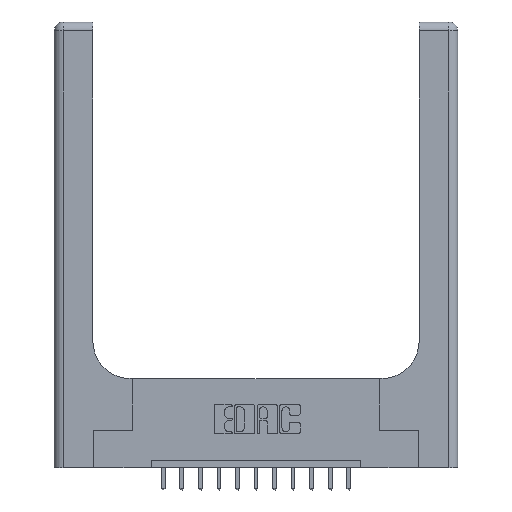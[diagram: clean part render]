
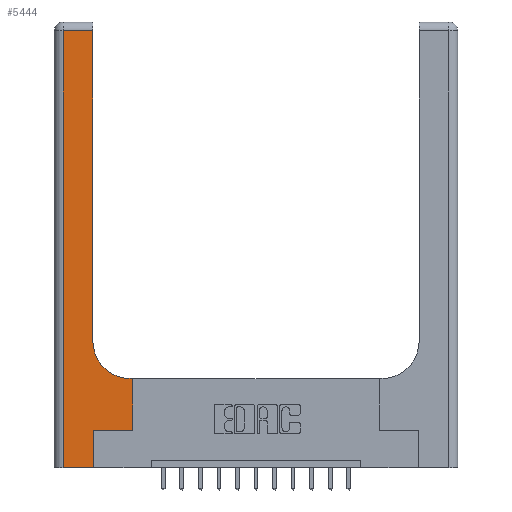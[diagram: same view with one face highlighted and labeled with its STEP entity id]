
A CAD part, top view. The second image highlights one B-rep face of the part: STEP entity #5444.
In plain terms, the highlighted planar face has unit normal (0, 0, 1).
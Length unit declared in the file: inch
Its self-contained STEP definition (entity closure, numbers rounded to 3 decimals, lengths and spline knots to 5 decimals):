
#220 = CARTESIAN_POINT ( 'NONE',  ( 0.51, 0.85, 0.37 ) ) ;
#249 = LINE ( 'NONE', #14911, #7896 ) ;
#260 = DIRECTION ( 'NONE',  ( 0., -1., 0. ) ) ;
#289 = VECTOR ( 'NONE', #5179, 39.37008 ) ;
#302 = DIRECTION ( 'NONE',  ( 0., 0., -1. ) ) ;
#724 = EDGE_CURVE ( 'NONE', #6429, #13446, #13874, .T. ) ;
#1127 = VERTEX_POINT ( 'NONE', #4149 ) ;
#1503 = VECTOR ( 'NONE', #8456, 39.37008 ) ;
#1571 = CARTESIAN_POINT ( 'NONE',  ( 0.528, 0.25, 0.37 ) ) ;
#1574 = CARTESIAN_POINT ( 'NONE',  ( 0.06, 0., 0.37 ) ) ;
#1593 = DIRECTION ( 'NONE',  ( 0., 0., -1. ) ) ;
#1599 = ORIENTED_EDGE ( 'NONE', *, *, #724, .T. ) ;
#1670 = FACE_OUTER_BOUND ( 'NONE', #6649, .T. ) ;
#1746 = VECTOR ( 'NONE', #3980, 39.37008 ) ;
#2108 = EDGE_CURVE ( 'NONE', #6239, #6429, #3733, .T. ) ;
#2227 = CARTESIAN_POINT ( 'NONE',  ( 0., 0., 0.37 ) ) ;
#2415 = VECTOR ( 'NONE', #10164, 39.37008 ) ;
#2502 = CARTESIAN_POINT ( 'NONE',  ( 0.26, 0.85, 0.37 ) ) ;
#2815 = VECTOR ( 'NONE', #260, 39.37008 ) ;
#3072 = DIRECTION ( 'NONE',  ( 1., 0., 0. ) ) ;
#3111 = DIRECTION ( 'NONE',  ( -1., 0., 0. ) ) ;
#3733 = LINE ( 'NONE', #10116, #4540 ) ;
#3980 = DIRECTION ( 'NONE',  ( 1., 0., 0. ) ) ;
#3993 = EDGE_CURVE ( 'NONE', #7947, #6239, #6394, .T. ) ;
#4127 = VERTEX_POINT ( 'NONE', #6884 ) ;
#4149 = CARTESIAN_POINT ( 'NONE',  ( 0.51, 0.6, 0.37 ) ) ;
#4290 = PLANE ( 'NONE',  #7903 ) ;
#4540 = VECTOR ( 'NONE', #7610, 39.37008 ) ;
#5090 = ORIENTED_EDGE ( 'NONE', *, *, #14723, .T. ) ;
#5179 = DIRECTION ( 'NONE',  ( 0., 1., 0. ) ) ;
#5444 = ADVANCED_FACE ( 'NONE', ( #1670 ), #4290, .F. ) ;
#5462 = EDGE_CURVE ( 'NONE', #8586, #14287, #6637, .T. ) ;
#5577 = DIRECTION ( 'NONE',  ( 0., 1., 0. ) ) ;
#5618 = ORIENTED_EDGE ( 'NONE', *, *, #2108, .T. ) ;
#6239 = VERTEX_POINT ( 'NONE', #7311 ) ;
#6394 = LINE ( 'NONE', #15412, #2415 ) ;
#6429 = VERTEX_POINT ( 'NONE', #1571 ) ;
#6637 = LINE ( 'NONE', #6725, #2815 ) ;
#6649 = EDGE_LOOP ( 'NONE', ( #9048, #15503, #15206, #15675, #10829, #5618, #1599, #8848, #5090 ) ) ;
#6706 = EDGE_CURVE ( 'NONE', #4127, #8586, #7115, .T. ) ;
#6725 = CARTESIAN_POINT ( 'NONE',  ( 0.06, 3., 0.37 ) ) ;
#6884 = CARTESIAN_POINT ( 'NONE',  ( 0.26, 2.94, 0.37 ) ) ;
#7115 = LINE ( 'NONE', #11091, #1503 ) ;
#7143 = AXIS2_PLACEMENT_3D ( 'NONE', #220, #302, #3072 ) ;
#7311 = CARTESIAN_POINT ( 'NONE',  ( 0.265, 0.25, 0.37 ) ) ;
#7610 = DIRECTION ( 'NONE',  ( 1., 0., 0. ) ) ;
#7896 = VECTOR ( 'NONE', #12388, 39.37008 ) ;
#7903 = AXIS2_PLACEMENT_3D ( 'NONE', #10757, #1593, #3111 ) ;
#7947 = VERTEX_POINT ( 'NONE', #16629 ) ;
#8456 = DIRECTION ( 'NONE',  ( -1., 0., 0. ) ) ;
#8586 = VERTEX_POINT ( 'NONE', #12579 ) ;
#8607 = LINE ( 'NONE', #2227, #1746 ) ;
#8848 = ORIENTED_EDGE ( 'NONE', *, *, #11208, .T. ) ;
#9048 = ORIENTED_EDGE ( 'NONE', *, *, #16165, .T. ) ;
#10116 = CARTESIAN_POINT ( 'NONE',  ( 0.265, 0.25, 0.37 ) ) ;
#10164 = DIRECTION ( 'NONE',  ( 0., 1., 0. ) ) ;
#10443 = LINE ( 'NONE', #11980, #14202 ) ;
#10630 = CIRCLE ( 'NONE', #7143, 0.25 ) ;
#10757 = CARTESIAN_POINT ( 'NONE',  ( 0., 3., 0.37 ) ) ;
#10829 = ORIENTED_EDGE ( 'NONE', *, *, #3993, .T. ) ;
#11091 = CARTESIAN_POINT ( 'NONE',  ( 0., 2.94, 0.37 ) ) ;
#11208 = EDGE_CURVE ( 'NONE', #13446, #1127, #249, .T. ) ;
#11594 = CARTESIAN_POINT ( 'NONE',  ( 0.528, 0.25, 0.37 ) ) ;
#11944 = EDGE_CURVE ( 'NONE', #14287, #7947, #8607, .T. ) ;
#11980 = CARTESIAN_POINT ( 'NONE',  ( 0.26, 3., 0.37 ) ) ;
#12388 = DIRECTION ( 'NONE',  ( -1., 0., 0. ) ) ;
#12579 = CARTESIAN_POINT ( 'NONE',  ( 0.06, 2.94, 0.37 ) ) ;
#12786 = VERTEX_POINT ( 'NONE', #2502 ) ;
#13446 = VERTEX_POINT ( 'NONE', #13599 ) ;
#13599 = CARTESIAN_POINT ( 'NONE',  ( 0.528, 0.6, 0.37 ) ) ;
#13874 = LINE ( 'NONE', #11594, #289 ) ;
#14202 = VECTOR ( 'NONE', #5577, 39.37008 ) ;
#14287 = VERTEX_POINT ( 'NONE', #1574 ) ;
#14723 = EDGE_CURVE ( 'NONE', #1127, #12786, #10630, .T. ) ;
#14911 = CARTESIAN_POINT ( 'NONE',  ( 0.26, 0.6, 0.37 ) ) ;
#15206 = ORIENTED_EDGE ( 'NONE', *, *, #5462, .T. ) ;
#15412 = CARTESIAN_POINT ( 'NONE',  ( 0.265, 0., 0.37 ) ) ;
#15503 = ORIENTED_EDGE ( 'NONE', *, *, #6706, .T. ) ;
#15675 = ORIENTED_EDGE ( 'NONE', *, *, #11944, .T. ) ;
#16165 = EDGE_CURVE ( 'NONE', #12786, #4127, #10443, .T. ) ;
#16629 = CARTESIAN_POINT ( 'NONE',  ( 0.265, 0., 0.37 ) ) ;
